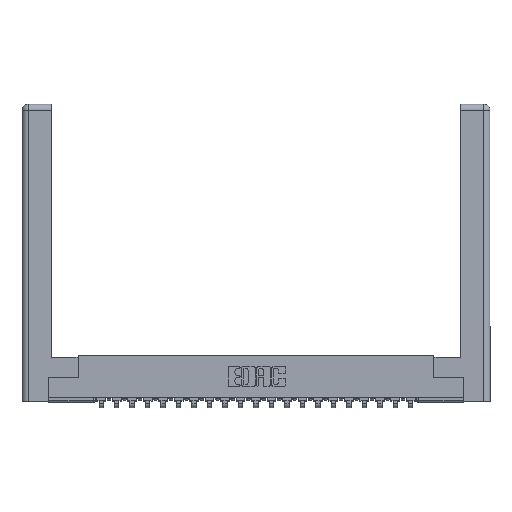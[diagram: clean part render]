
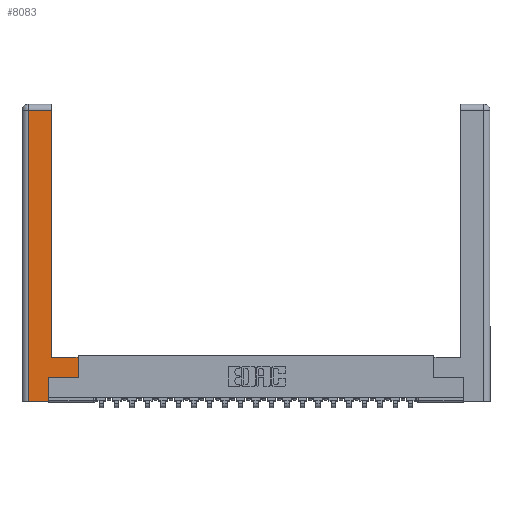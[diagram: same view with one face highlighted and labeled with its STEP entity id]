
A CAD part, top view. The second image highlights one B-rep face of the part: STEP entity #8083.
In plain terms, the highlighted planar face has unit normal (0, 0, 1).
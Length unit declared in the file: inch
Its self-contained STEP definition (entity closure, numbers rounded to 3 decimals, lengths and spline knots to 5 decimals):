
#526 = LINE ( 'NONE', #5650, #10396 ) ;
#1058 = VECTOR ( 'NONE', #2191, 39.37008 ) ;
#1641 = CARTESIAN_POINT ( 'NONE',  ( 0.295, 3., 0. ) ) ;
#1837 = DIRECTION ( 'NONE',  ( 0., 0., -1. ) ) ;
#1964 = VERTEX_POINT ( 'NONE', #3373 ) ;
#2191 = DIRECTION ( 'NONE',  ( 0., -1., 0. ) ) ;
#2736 = ORIENTED_EDGE ( 'NONE', *, *, #19817, .T. ) ;
#3124 = CARTESIAN_POINT ( 'NONE',  ( 0.0615, 2.94, 0. ) ) ;
#3270 = EDGE_CURVE ( 'NONE', #6939, #15283, #526, .T. ) ;
#3373 = CARTESIAN_POINT ( 'NONE',  ( 0.565, 0.45, 0. ) ) ;
#3506 = CARTESIAN_POINT ( 'NONE',  ( 0.265, 0., 0. ) ) ;
#3857 = CARTESIAN_POINT ( 'NONE',  ( 0.565, 0.245, 0. ) ) ;
#4452 = EDGE_CURVE ( 'NONE', #17155, #16565, #20805, .T. ) ;
#5650 = CARTESIAN_POINT ( 'NONE',  ( 0.565, 0.245, 0. ) ) ;
#5695 = EDGE_CURVE ( 'NONE', #1964, #10917, #7479, .T. ) ;
#6412 = ORIENTED_EDGE ( 'NONE', *, *, #5695, .T. ) ;
#6939 = VERTEX_POINT ( 'NONE', #22694 ) ;
#7479 = LINE ( 'NONE', #16056, #9986 ) ;
#7906 = LINE ( 'NONE', #11931, #13442 ) ;
#8068 = LINE ( 'NONE', #12821, #20556 ) ;
#8083 = ADVANCED_FACE ( 'NONE', ( #16869 ), #18489, .F. ) ;
#8614 = VERTEX_POINT ( 'NONE', #3506 ) ;
#8653 = CARTESIAN_POINT ( 'NONE',  ( 0.265, 0., 0. ) ) ;
#8742 = DIRECTION ( 'NONE',  ( -1., 0., 0. ) ) ;
#9077 = ORIENTED_EDGE ( 'NONE', *, *, #16904, .T. ) ;
#9159 = VECTOR ( 'NONE', #21646, 39.37008 ) ;
#9986 = VECTOR ( 'NONE', #8742, 39.37008 ) ;
#10278 = EDGE_CURVE ( 'NONE', #10917, #15262, #23753, .T. ) ;
#10360 = LINE ( 'NONE', #10904, #17924 ) ;
#10396 = VECTOR ( 'NONE', #15002, 39.37008 ) ;
#10904 = CARTESIAN_POINT ( 'NONE',  ( 0.0615, 2.94, 0. ) ) ;
#10917 = VERTEX_POINT ( 'NONE', #20209 ) ;
#11694 = CARTESIAN_POINT ( 'NONE',  ( 0.0615, 0., 0. ) ) ;
#11931 = CARTESIAN_POINT ( 'NONE',  ( 0.565, 0.45, 0. ) ) ;
#12376 = AXIS2_PLACEMENT_3D ( 'NONE', #12962, #1837, #14840 ) ;
#12821 = CARTESIAN_POINT ( 'NONE',  ( 0.265, 0.245, 0. ) ) ;
#12962 = CARTESIAN_POINT ( 'NONE',  ( 0., 0., 0. ) ) ;
#13442 = VECTOR ( 'NONE', #19396, 39.37008 ) ;
#14778 = CARTESIAN_POINT ( 'NONE',  ( 0.0615, 0., 0. ) ) ;
#14840 = DIRECTION ( 'NONE',  ( -1., 0., 0. ) ) ;
#15002 = DIRECTION ( 'NONE',  ( 1., 0., 0. ) ) ;
#15262 = VERTEX_POINT ( 'NONE', #18237 ) ;
#15283 = VERTEX_POINT ( 'NONE', #3857 ) ;
#16056 = CARTESIAN_POINT ( 'NONE',  ( 0.295, 0.45, 0. ) ) ;
#16565 = VERTEX_POINT ( 'NONE', #14778 ) ;
#16786 = VECTOR ( 'NONE', #20236, 39.37008 ) ;
#16869 = FACE_OUTER_BOUND ( 'NONE', #21280, .T. ) ;
#16904 = EDGE_CURVE ( 'NONE', #15283, #1964, #7906, .T. ) ;
#17155 = VERTEX_POINT ( 'NONE', #3124 ) ;
#17893 = LINE ( 'NONE', #8653, #9159 ) ;
#17924 = VECTOR ( 'NONE', #18462, 39.37008 ) ;
#17989 = ORIENTED_EDGE ( 'NONE', *, *, #3270, .T. ) ;
#18237 = CARTESIAN_POINT ( 'NONE',  ( 0.295, 2.94, 0. ) ) ;
#18462 = DIRECTION ( 'NONE',  ( -1., 0., 0. ) ) ;
#18489 = PLANE ( 'NONE',  #12376 ) ;
#19396 = DIRECTION ( 'NONE',  ( 0., 1., 0. ) ) ;
#19817 = EDGE_CURVE ( 'NONE', #8614, #6939, #8068, .T. ) ;
#20025 = ORIENTED_EDGE ( 'NONE', *, *, #20162, .T. ) ;
#20162 = EDGE_CURVE ( 'NONE', #15262, #17155, #10360, .T. ) ;
#20209 = CARTESIAN_POINT ( 'NONE',  ( 0.295, 0.45, 0. ) ) ;
#20236 = DIRECTION ( 'NONE',  ( 0., 1., 0. ) ) ;
#20556 = VECTOR ( 'NONE', #22250, 39.37008 ) ;
#20805 = LINE ( 'NONE', #11694, #1058 ) ;
#21231 = ORIENTED_EDGE ( 'NONE', *, *, #4452, .T. ) ;
#21264 = EDGE_CURVE ( 'NONE', #16565, #8614, #17893, .T. ) ;
#21280 = EDGE_LOOP ( 'NONE', ( #23180, #20025, #21231, #23359, #2736, #17989, #9077, #6412 ) ) ;
#21646 = DIRECTION ( 'NONE',  ( 1., 0., 0. ) ) ;
#22250 = DIRECTION ( 'NONE',  ( 0., 1., 0. ) ) ;
#22694 = CARTESIAN_POINT ( 'NONE',  ( 0.265, 0.245, 0. ) ) ;
#23180 = ORIENTED_EDGE ( 'NONE', *, *, #10278, .T. ) ;
#23359 = ORIENTED_EDGE ( 'NONE', *, *, #21264, .T. ) ;
#23753 = LINE ( 'NONE', #1641, #16786 ) ;
